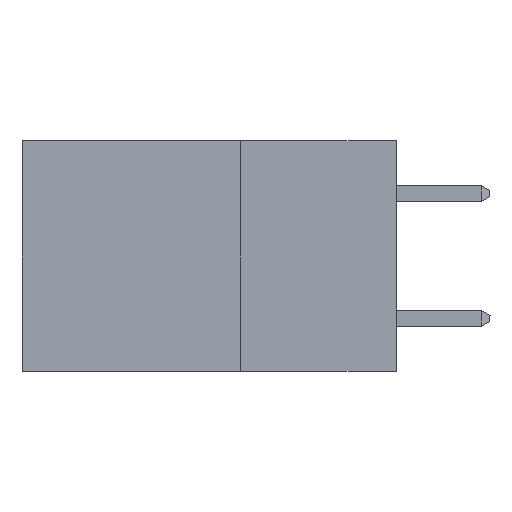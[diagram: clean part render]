
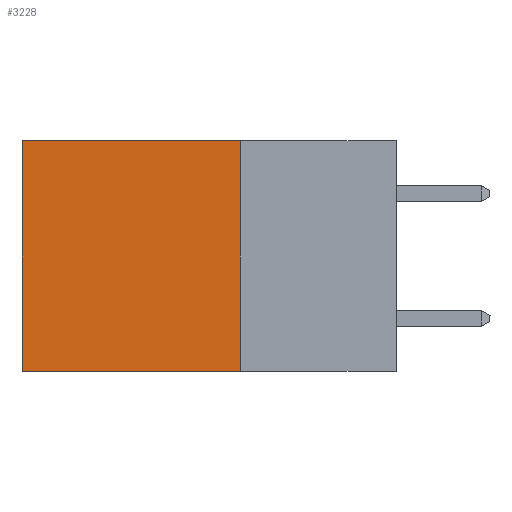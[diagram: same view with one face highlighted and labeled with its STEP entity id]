
A CAD part, left-side view. The second image highlights one B-rep face of the part: STEP entity #3228.
In plain terms, the highlighted planar face has unit normal (-1, 0, 0).
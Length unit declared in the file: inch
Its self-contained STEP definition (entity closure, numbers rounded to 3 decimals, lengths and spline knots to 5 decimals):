
#750 = DIRECTION ( 'NONE',  ( 0., 0., -1. ) ) ;
#3023 = VERTEX_POINT ( 'NONE', #6423 ) ;
#3228 = ADVANCED_FACE ( 'NONE', ( #5468 ), #7325, .F. ) ;
#3939 = ORIENTED_EDGE ( 'NONE', *, *, #14080, .T. ) ;
#4112 = LINE ( 'NONE', #4566, #10292 ) ;
#4129 = DIRECTION ( 'NONE',  ( 0., 0., -1. ) ) ;
#4135 = CARTESIAN_POINT ( 'NONE',  ( 0.2615, 0.25, -0.37 ) ) ;
#4477 = VECTOR ( 'NONE', #6955, 39.37008 ) ;
#4566 = CARTESIAN_POINT ( 'NONE',  ( 0.2615, 0.6, -0.37 ) ) ;
#4775 = CARTESIAN_POINT ( 'NONE',  ( 0.2615, 0.25, 0. ) ) ;
#4855 = LINE ( 'NONE', #7017, #4477 ) ;
#4924 = EDGE_CURVE ( 'NONE', #12043, #12283, #14367, .T. ) ;
#5468 = FACE_OUTER_BOUND ( 'NONE', #11757, .T. ) ;
#6423 = CARTESIAN_POINT ( 'NONE',  ( 0.2615, 0.6, 0. ) ) ;
#6551 = EDGE_CURVE ( 'NONE', #12043, #3023, #8312, .T. ) ;
#6627 = DIRECTION ( 'NONE',  ( 1., 0., 0. ) ) ;
#6813 = VERTEX_POINT ( 'NONE', #8751 ) ;
#6955 = DIRECTION ( 'NONE',  ( 0., 1., 0. ) ) ;
#7017 = CARTESIAN_POINT ( 'NONE',  ( 0.2615, 0.25, -0.37 ) ) ;
#7056 = EDGE_CURVE ( 'NONE', #12283, #6813, #4855, .T. ) ;
#7156 = CARTESIAN_POINT ( 'NONE',  ( 0.2615, 0.25, -0.37 ) ) ;
#7318 = ORIENTED_EDGE ( 'NONE', *, *, #7056, .F. ) ;
#7325 = PLANE ( 'NONE',  #7569 ) ;
#7569 = AXIS2_PLACEMENT_3D ( 'NONE', #7156, #6627, #750 ) ;
#7729 = ORIENTED_EDGE ( 'NONE', *, *, #4924, .F. ) ;
#8312 = LINE ( 'NONE', #10896, #13987 ) ;
#8330 = VECTOR ( 'NONE', #4129, 39.37008 ) ;
#8629 = ORIENTED_EDGE ( 'NONE', *, *, #6551, .T. ) ;
#8751 = CARTESIAN_POINT ( 'NONE',  ( 0.2615, 0.6, -0.37 ) ) ;
#10292 = VECTOR ( 'NONE', #12592, 39.37008 ) ;
#10896 = CARTESIAN_POINT ( 'NONE',  ( 0.2615, 0.25, 0. ) ) ;
#10941 = DIRECTION ( 'NONE',  ( 0., 1., 0. ) ) ;
#11757 = EDGE_LOOP ( 'NONE', ( #3939, #7318, #7729, #8629 ) ) ;
#12043 = VERTEX_POINT ( 'NONE', #4775 ) ;
#12283 = VERTEX_POINT ( 'NONE', #14373 ) ;
#12592 = DIRECTION ( 'NONE',  ( 0., 0., -1. ) ) ;
#13987 = VECTOR ( 'NONE', #10941, 39.37008 ) ;
#14080 = EDGE_CURVE ( 'NONE', #3023, #6813, #4112, .T. ) ;
#14367 = LINE ( 'NONE', #4135, #8330 ) ;
#14373 = CARTESIAN_POINT ( 'NONE',  ( 0.2615, 0.25, -0.37 ) ) ;
